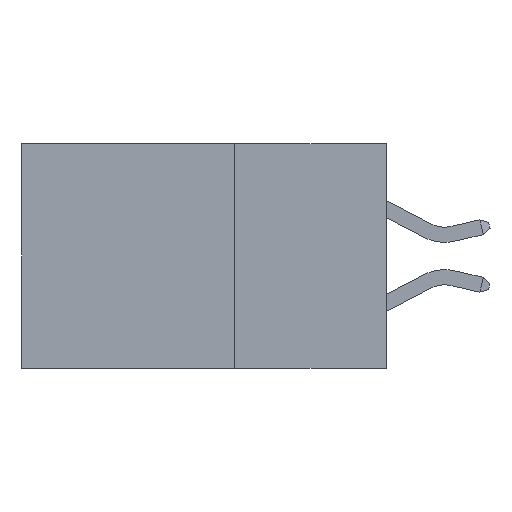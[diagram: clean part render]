
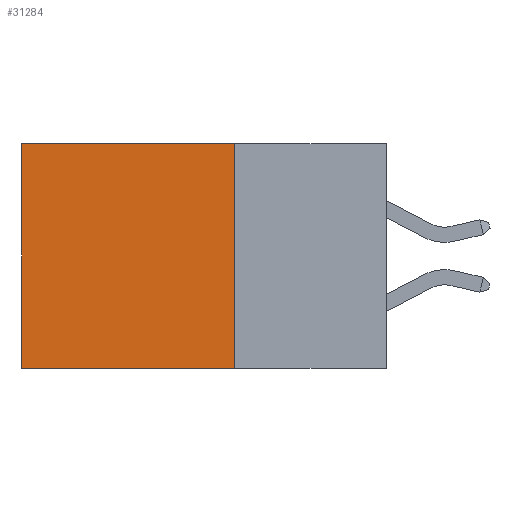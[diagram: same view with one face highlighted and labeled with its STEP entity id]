
A CAD part, left-side view. The second image highlights one B-rep face of the part: STEP entity #31284.
In plain terms, the highlighted planar face has unit normal (-1, 0, 0).
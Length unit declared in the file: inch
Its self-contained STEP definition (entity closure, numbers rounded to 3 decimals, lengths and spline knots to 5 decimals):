
#453 = EDGE_CURVE ( 'NONE', #21190, #16001, #3810, .T. ) ;
#1944 = CARTESIAN_POINT ( 'NONE',  ( 0.298, 0.25, -0.37 ) ) ;
#2254 = CARTESIAN_POINT ( 'NONE',  ( 0.298, 0.25, 0. ) ) ;
#2518 = CARTESIAN_POINT ( 'NONE',  ( 0.298, 0.6, 0. ) ) ;
#2637 = VECTOR ( 'NONE', #2941, 39.37008 ) ;
#2941 = DIRECTION ( 'NONE',  ( 0., 0., -1. ) ) ;
#3806 = PLANE ( 'NONE',  #17622 ) ;
#3810 = LINE ( 'NONE', #2518, #2637 ) ;
#6483 = DIRECTION ( 'NONE',  ( 1., 0., 0. ) ) ;
#6889 = ORIENTED_EDGE ( 'NONE', *, *, #12660, .T. ) ;
#6917 = DIRECTION ( 'NONE',  ( 0., 0., -1. ) ) ;
#7244 = EDGE_CURVE ( 'NONE', #7929, #14277, #20805, .T. ) ;
#7929 = VERTEX_POINT ( 'NONE', #2254 ) ;
#8073 = DIRECTION ( 'NONE',  ( 0., 0., -1. ) ) ;
#8355 = LINE ( 'NONE', #10346, #18220 ) ;
#9356 = VECTOR ( 'NONE', #8073, 39.37008 ) ;
#10346 = CARTESIAN_POINT ( 'NONE',  ( 0.298, 0.25, -0.37 ) ) ;
#10733 = CARTESIAN_POINT ( 'NONE',  ( 0.298, 0.25, 0. ) ) ;
#12660 = EDGE_CURVE ( 'NONE', #7929, #21190, #23960, .T. ) ;
#13833 = ORIENTED_EDGE ( 'NONE', *, *, #453, .T. ) ;
#14277 = VERTEX_POINT ( 'NONE', #1944 ) ;
#16001 = VERTEX_POINT ( 'NONE', #20548 ) ;
#16793 = EDGE_CURVE ( 'NONE', #14277, #16001, #8355, .T. ) ;
#17070 = CARTESIAN_POINT ( 'NONE',  ( 0.298, 0.25, 0. ) ) ;
#17280 = VECTOR ( 'NONE', #22022, 39.37008 ) ;
#17492 = FACE_OUTER_BOUND ( 'NONE', #18550, .T. ) ;
#17622 = AXIS2_PLACEMENT_3D ( 'NONE', #31637, #6483, #6917 ) ;
#18220 = VECTOR ( 'NONE', #20575, 39.37008 ) ;
#18550 = EDGE_LOOP ( 'NONE', ( #13833, #21470, #29954, #6889 ) ) ;
#20222 = CARTESIAN_POINT ( 'NONE',  ( 0.298, 0.6, 0. ) ) ;
#20548 = CARTESIAN_POINT ( 'NONE',  ( 0.298, 0.6, -0.37 ) ) ;
#20575 = DIRECTION ( 'NONE',  ( 0., 1., 0. ) ) ;
#20805 = LINE ( 'NONE', #10733, #9356 ) ;
#21190 = VERTEX_POINT ( 'NONE', #20222 ) ;
#21470 = ORIENTED_EDGE ( 'NONE', *, *, #16793, .F. ) ;
#22022 = DIRECTION ( 'NONE',  ( 0., 1., 0. ) ) ;
#23960 = LINE ( 'NONE', #17070, #17280 ) ;
#29954 = ORIENTED_EDGE ( 'NONE', *, *, #7244, .F. ) ;
#31284 = ADVANCED_FACE ( 'NONE', ( #17492 ), #3806, .F. ) ;
#31637 = CARTESIAN_POINT ( 'NONE',  ( 0.298, 0.25, 0. ) ) ;
